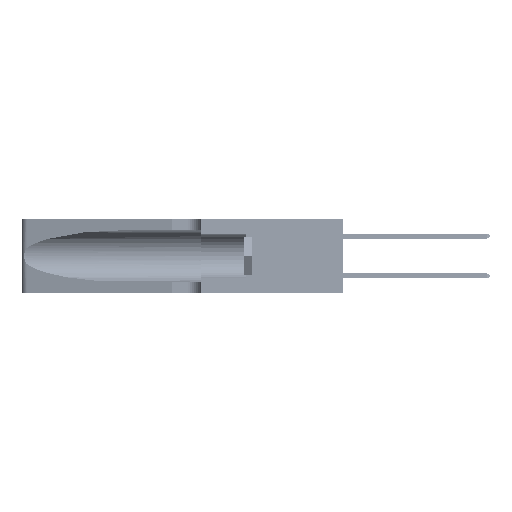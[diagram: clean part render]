
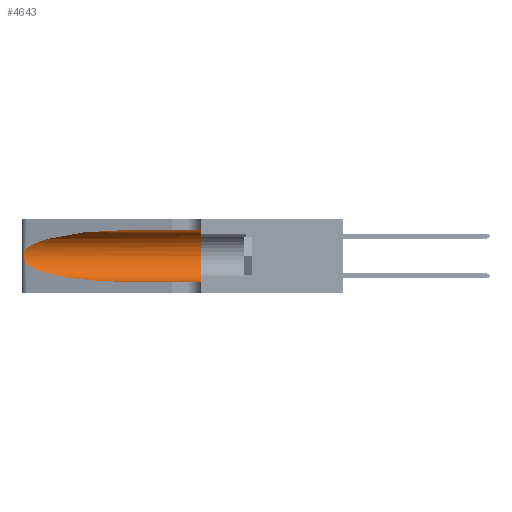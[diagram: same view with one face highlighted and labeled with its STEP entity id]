
A CAD part, left-side view. The second image highlights one B-rep face of the part: STEP entity #4643.
In plain terms, the highlighted cylindrical face has radius 3.308 mm (diameter 6.617 mm), a partial arc.
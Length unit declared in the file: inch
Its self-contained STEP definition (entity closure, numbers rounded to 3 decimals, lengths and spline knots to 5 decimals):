
#251 = CARTESIAN_POINT ( 'NONE',  ( 0.25854, 1.2359, 0.20912 ) ) ;
#1749 = FACE_OUTER_BOUND ( 'NONE', #18427, .T. ) ;
#3388 = ORIENTED_EDGE ( 'NONE', *, *, #45652, .T. ) ;
#4110 = LINE ( 'NONE', #37946, #23506 ) ;
#4643 = ADVANCED_FACE ( 'NONE', ( #1749 ), #44839, .F. ) ;
#4661 = DIRECTION ( 'NONE',  ( 0., -1., 0. ) ) ;
#4813 = EDGE_CURVE ( 'NONE', #19394, #9340, #13284, .T. ) ;
#4984 = ORIENTED_EDGE ( 'NONE', *, *, #11407, .T. ) ;
#6910 = DIRECTION ( 'NONE',  ( 0., -1., 0. ) ) ;
#7577 = ORIENTED_EDGE ( 'NONE', *, *, #17315, .F. ) ;
#7905 = CARTESIAN_POINT ( 'NONE',  ( 0.25789, 1.23486, 0.15765 ) ) ;
#8068 = CARTESIAN_POINT ( 'NONE',  ( 0.25555, 1.22993, 0.14849 ) ) ;
#9340 = VERTEX_POINT ( 'NONE', #38932 ) ;
#9743 = ORIENTED_EDGE ( 'NONE', *, *, #32580, .T. ) ;
#11407 = EDGE_CURVE ( 'NONE', #26235, #21938, #15030, .T. ) ;
#12453 = DIRECTION ( 'NONE',  ( 0., 0., -1. ) ) ;
#13284 = CIRCLE ( 'NONE', #28548, 0.13025 ) ;
#13559 = DIRECTION ( 'NONE',  ( 0., -1., 0. ) ) ;
#15030 =( BOUNDED_CURVE ( )  B_SPLINE_CURVE ( 3, ( #32783, #36692, #21218, #36187 ),
 .UNSPECIFIED., .F., .F. ) 
 B_SPLINE_CURVE_WITH_KNOTS ( ( 4, 4 ),
 ( 3.44316, 4.71239 ),
 .UNSPECIFIED. ) 
 CURVE ( )  GEOMETRIC_REPRESENTATION_ITEM ( )  RATIONAL_B_SPLINE_CURVE ( ( 1., 0.87, 0.87, 1. ) ) 
 REPRESENTATION_ITEM ( '' )  );
#15359 = CARTESIAN_POINT ( 'NONE',  ( 0.25487, 1.22718, 0.22369 ) ) ;
#15870 = CARTESIAN_POINT ( 'NONE',  ( 0.26017, 1.23833, 0.17102 ) ) ;
#16198 = CARTESIAN_POINT ( 'NONE',  ( 0.25787, 1.23484, 0.2124 ) ) ;
#17315 = EDGE_CURVE ( 'NONE', #18257, #19394, #4110, .T. ) ;
#18053 = CARTESIAN_POINT ( 'NONE',  ( 0.1305, 0.35, 0.185 ) ) ;
#18257 = VERTEX_POINT ( 'NONE', #23330 ) ;
#18427 = EDGE_LOOP ( 'NONE', ( #3388, #41461, #4984, #9743, #27721, #7577 ) ) ;
#19189 = CARTESIAN_POINT ( 'NONE',  ( 0.1305, 0.72297, 0.31525 ) ) ;
#19394 = VERTEX_POINT ( 'NONE', #26138 ) ;
#20050 = CARTESIAN_POINT ( 'NONE',  ( 0.26018, 1.23835, 0.19895 ) ) ;
#21218 = CARTESIAN_POINT ( 'NONE',  ( 0.18966, 0.96281, 0.05475 ) ) ;
#21938 = VERTEX_POINT ( 'NONE', #37179 ) ;
#22443 =( BOUNDED_CURVE ( )  B_SPLINE_CURVE ( 3, ( #19189, #27032, #34157, #15359 ),
 .UNSPECIFIED., .F., .F. ) 
 B_SPLINE_CURVE_WITH_KNOTS ( ( 4, 4 ),
 ( 1.5708, 2.84003 ),
 .UNSPECIFIED. ) 
 CURVE ( )  GEOMETRIC_REPRESENTATION_ITEM ( )  RATIONAL_B_SPLINE_CURVE ( ( 1., 0.87, 0.87, 1. ) ) 
 REPRESENTATION_ITEM ( '' )  );
#23330 = CARTESIAN_POINT ( 'NONE',  ( 0.1305, 0.72297, 0.31525 ) ) ;
#23506 = VECTOR ( 'NONE', #6910, 39.37008 ) ;
#26138 = CARTESIAN_POINT ( 'NONE',  ( 0.1305, 0.35, 0.31525 ) ) ;
#26235 = VERTEX_POINT ( 'NONE', #48485 ) ;
#26458 = CARTESIAN_POINT ( 'NONE',  ( 0.25555, 1.22994, 0.2215 ) ) ;
#27032 = CARTESIAN_POINT ( 'NONE',  ( 0.18966, 0.96281, 0.31525 ) ) ;
#27401 = CARTESIAN_POINT ( 'NONE',  ( 0.25639, 1.23186, 0.15144 ) ) ;
#27721 = ORIENTED_EDGE ( 'NONE', *, *, #4813, .F. ) ;
#27727 = CARTESIAN_POINT ( 'NONE',  ( 0.26075, 1.23896, 0.178 ) ) ;
#28548 = AXIS2_PLACEMENT_3D ( 'NONE', #18053, #36920, #45527 ) ;
#31270 = CARTESIAN_POINT ( 'NONE',  ( 0.25639, 1.23184, 0.21858 ) ) ;
#32580 = EDGE_CURVE ( 'NONE', #21938, #9340, #42446, .T. ) ;
#32783 = CARTESIAN_POINT ( 'NONE',  ( 0.25487, 1.22718, 0.14631 ) ) ;
#34081 = CARTESIAN_POINT ( 'NONE',  ( 0.25487, 1.22718, 0.22369 ) ) ;
#34157 = CARTESIAN_POINT ( 'NONE',  ( 0.2373, 1.15595, 0.28018 ) ) ;
#35342 = CARTESIAN_POINT ( 'NONE',  ( 0.26075, 1.23896, 0.19203 ) ) ;
#35832 = B_SPLINE_CURVE_WITH_KNOTS ( 'NONE', 3,
 ( #34081, #26458, #31270, #16198, #251, #20050, #35342, #27727, #15870, #47216, #7905, #27401, #8068, #46885 ),
 .UNSPECIFIED., .F., .F.,
 ( 4, 2, 2, 2, 2, 2, 4 ),
 ( 0., 0.00027, 0.00053, 0.00107, 0.0016, 0.00187, 0.00214 ),
 .UNSPECIFIED. ) ;
#36187 = CARTESIAN_POINT ( 'NONE',  ( 0.1305, 0.72297, 0.05475 ) ) ;
#36692 = CARTESIAN_POINT ( 'NONE',  ( 0.2373, 1.15595, 0.08982 ) ) ;
#36920 = DIRECTION ( 'NONE',  ( 0., 1., 0. ) ) ;
#37179 = CARTESIAN_POINT ( 'NONE',  ( 0.1305, 0.72297, 0.05475 ) ) ;
#37946 = CARTESIAN_POINT ( 'NONE',  ( 0.1305, 1.61858, 0.31525 ) ) ;
#38152 = CARTESIAN_POINT ( 'NONE',  ( 0.25487, 1.22718, 0.22369 ) ) ;
#38932 = CARTESIAN_POINT ( 'NONE',  ( 0.1305, 0.35, 0.05475 ) ) ;
#39774 = CARTESIAN_POINT ( 'NONE',  ( 0.1305, 1.61858, 0.185 ) ) ;
#41461 = ORIENTED_EDGE ( 'NONE', *, *, #42910, .T. ) ;
#42446 = LINE ( 'NONE', #43917, #43016 ) ;
#42804 = VERTEX_POINT ( 'NONE', #38152 ) ;
#42910 = EDGE_CURVE ( 'NONE', #42804, #26235, #35832, .T. ) ;
#43016 = VECTOR ( 'NONE', #13559, 39.37008 ) ;
#43917 = CARTESIAN_POINT ( 'NONE',  ( 0.1305, 1.61858, 0.05475 ) ) ;
#44150 = AXIS2_PLACEMENT_3D ( 'NONE', #39774, #4661, #12453 ) ;
#44839 = CYLINDRICAL_SURFACE ( 'NONE', #44150, 0.13025 ) ;
#45527 = DIRECTION ( 'NONE',  ( 0., 0., 1. ) ) ;
#45652 = EDGE_CURVE ( 'NONE', #18257, #42804, #22443, .T. ) ;
#46885 = CARTESIAN_POINT ( 'NONE',  ( 0.25487, 1.22718, 0.14631 ) ) ;
#47216 = CARTESIAN_POINT ( 'NONE',  ( 0.25856, 1.23593, 0.16098 ) ) ;
#48485 = CARTESIAN_POINT ( 'NONE',  ( 0.25487, 1.22718, 0.14631 ) ) ;
